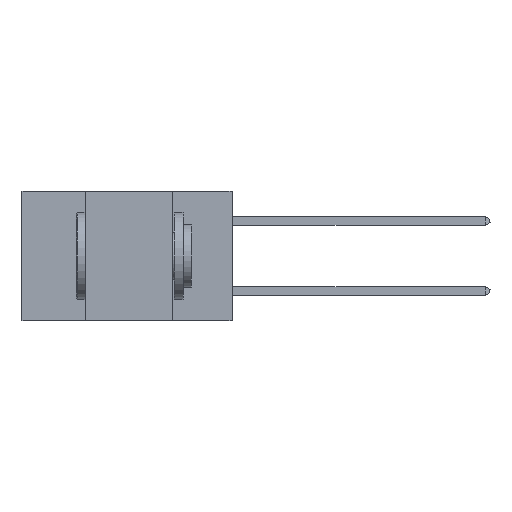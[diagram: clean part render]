
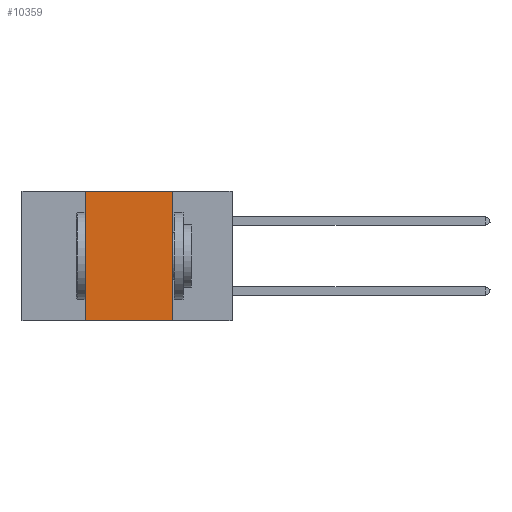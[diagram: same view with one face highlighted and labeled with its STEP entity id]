
A CAD part, left-side view. The second image highlights one B-rep face of the part: STEP entity #10359.
In plain terms, the highlighted planar face has unit normal (-1, 0, 0).
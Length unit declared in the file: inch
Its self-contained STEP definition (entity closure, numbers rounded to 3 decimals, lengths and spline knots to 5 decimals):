
#172 = ORIENTED_EDGE ( 'NONE', *, *, #35264, .F. ) ;
#2492 = EDGE_CURVE ( 'NONE', #25525, #10285, #15730, .T. ) ;
#2911 = FACE_OUTER_BOUND ( 'NONE', #11127, .T. ) ;
#3842 = DIRECTION ( 'NONE',  ( 0., 0., -1. ) ) ;
#4217 = VECTOR ( 'NONE', #10168, 39.37008 ) ;
#6746 = CARTESIAN_POINT ( 'NONE',  ( 0., 0.17, 0. ) ) ;
#6934 = ORIENTED_EDGE ( 'NONE', *, *, #23318, .F. ) ;
#7054 = VECTOR ( 'NONE', #14516, 39.37008 ) ;
#9807 = AXIS2_PLACEMENT_3D ( 'NONE', #30933, #12143, #18455 ) ;
#10168 = DIRECTION ( 'NONE',  ( 0., 0., 1. ) ) ;
#10285 = VERTEX_POINT ( 'NONE', #27791 ) ;
#10359 = ADVANCED_FACE ( 'NONE', ( #2911 ), #21449, .F. ) ;
#11088 = CARTESIAN_POINT ( 'NONE',  ( 0., 0.42, -0.37 ) ) ;
#11127 = EDGE_LOOP ( 'NONE', ( #6934, #34370, #172, #22470 ) ) ;
#12143 = DIRECTION ( 'NONE',  ( 1., 0., 0. ) ) ;
#13608 = CARTESIAN_POINT ( 'NONE',  ( 0., 0.42, 0. ) ) ;
#14516 = DIRECTION ( 'NONE',  ( 0., -1., 0. ) ) ;
#14828 = EDGE_CURVE ( 'NONE', #22151, #23952, #23747, .T. ) ;
#15475 = DIRECTION ( 'NONE',  ( 0., -1., 0. ) ) ;
#15730 = LINE ( 'NONE', #18478, #27449 ) ;
#16271 = VECTOR ( 'NONE', #3842, 39.37008 ) ;
#16600 = CARTESIAN_POINT ( 'NONE',  ( 0., 0.42, 0. ) ) ;
#18455 = DIRECTION ( 'NONE',  ( 0., 0., -1. ) ) ;
#18478 = CARTESIAN_POINT ( 'NONE',  ( 0., 0.6, 0. ) ) ;
#20085 = CARTESIAN_POINT ( 'NONE',  ( 0., 0.17, -0.37 ) ) ;
#21449 = PLANE ( 'NONE',  #9807 ) ;
#22151 = VERTEX_POINT ( 'NONE', #11088 ) ;
#22470 = ORIENTED_EDGE ( 'NONE', *, *, #14828, .T. ) ;
#23318 = EDGE_CURVE ( 'NONE', #10285, #23952, #24600, .T. ) ;
#23747 = LINE ( 'NONE', #27263, #7054 ) ;
#23952 = VERTEX_POINT ( 'NONE', #20085 ) ;
#24600 = LINE ( 'NONE', #6746, #16271 ) ;
#25525 = VERTEX_POINT ( 'NONE', #13608 ) ;
#27263 = CARTESIAN_POINT ( 'NONE',  ( 0., 0.6, -0.37 ) ) ;
#27449 = VECTOR ( 'NONE', #15475, 39.37008 ) ;
#27791 = CARTESIAN_POINT ( 'NONE',  ( 0., 0.17, 0. ) ) ;
#29271 = LINE ( 'NONE', #16600, #4217 ) ;
#30933 = CARTESIAN_POINT ( 'NONE',  ( 0., 0.6, 0. ) ) ;
#34370 = ORIENTED_EDGE ( 'NONE', *, *, #2492, .F. ) ;
#35264 = EDGE_CURVE ( 'NONE', #22151, #25525, #29271, .T. ) ;
